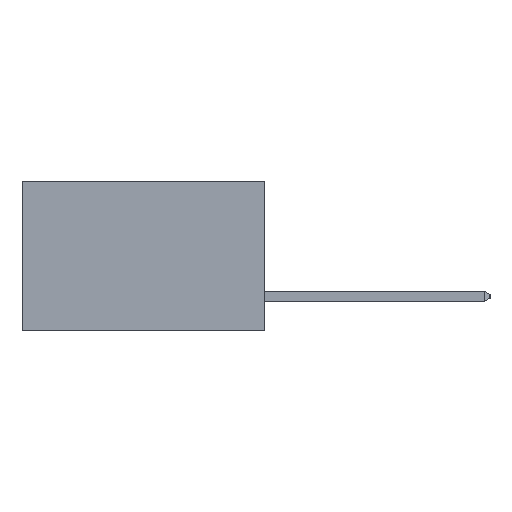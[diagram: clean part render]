
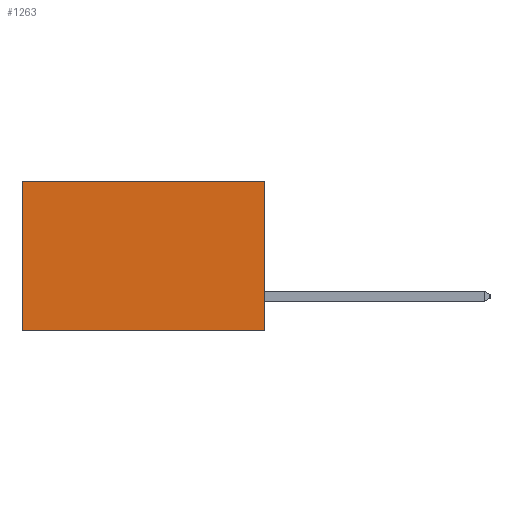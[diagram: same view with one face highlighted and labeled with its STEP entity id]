
A CAD part, left-side view. The second image highlights one B-rep face of the part: STEP entity #1263.
In plain terms, the highlighted planar face has unit normal (-1, 0, 0).
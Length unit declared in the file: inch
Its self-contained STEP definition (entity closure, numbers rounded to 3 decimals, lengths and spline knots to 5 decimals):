
#1263 = ADVANCED_FACE ( 'NONE', ( #21789 ), #15451, .F. ) ;
#1302 = EDGE_LOOP ( 'NONE', ( #18955, #6433, #19054, #21128 ) ) ;
#1307 = EDGE_CURVE ( 'NONE', #15340, #2263, #1640, .T. ) ;
#1640 = LINE ( 'NONE', #10880, #11262 ) ;
#1759 = CARTESIAN_POINT ( 'NONE',  ( 0.2615, 0.6, -0.37 ) ) ;
#2263 = VERTEX_POINT ( 'NONE', #3046 ) ;
#2740 = VECTOR ( 'NONE', #22175, 39.37008 ) ;
#3046 = CARTESIAN_POINT ( 'NONE',  ( 0.2615, 0.6, 0. ) ) ;
#3265 = CARTESIAN_POINT ( 'NONE',  ( 0.2615, 0.6, -0.37 ) ) ;
#4003 = LINE ( 'NONE', #20665, #22865 ) ;
#6433 = ORIENTED_EDGE ( 'NONE', *, *, #14882, .F. ) ;
#8589 = VECTOR ( 'NONE', #19528, 39.37008 ) ;
#10880 = CARTESIAN_POINT ( 'NONE',  ( 0.2615, 0., 0. ) ) ;
#10926 = CARTESIAN_POINT ( 'NONE',  ( 0.2615, 0., 0. ) ) ;
#11262 = VECTOR ( 'NONE', #13035, 39.37008 ) ;
#11428 = CARTESIAN_POINT ( 'NONE',  ( 0.2615, 0., -0.37 ) ) ;
#13035 = DIRECTION ( 'NONE',  ( 0., 1., 0. ) ) ;
#14216 = DIRECTION ( 'NONE',  ( 1., 0., 0. ) ) ;
#14882 = EDGE_CURVE ( 'NONE', #14916, #16942, #4003, .T. ) ;
#14916 = VERTEX_POINT ( 'NONE', #11428 ) ;
#15318 = EDGE_CURVE ( 'NONE', #2263, #16942, #22838, .T. ) ;
#15340 = VERTEX_POINT ( 'NONE', #10926 ) ;
#15451 = PLANE ( 'NONE',  #23862 ) ;
#16942 = VERTEX_POINT ( 'NONE', #1759 ) ;
#18955 = ORIENTED_EDGE ( 'NONE', *, *, #15318, .T. ) ;
#19035 = EDGE_CURVE ( 'NONE', #15340, #14916, #23472, .T. ) ;
#19054 = ORIENTED_EDGE ( 'NONE', *, *, #19035, .F. ) ;
#19089 = DIRECTION ( 'NONE',  ( 0., 0., -1. ) ) ;
#19528 = DIRECTION ( 'NONE',  ( 0., 0., -1. ) ) ;
#20665 = CARTESIAN_POINT ( 'NONE',  ( 0.2615, 0., -0.37 ) ) ;
#21128 = ORIENTED_EDGE ( 'NONE', *, *, #1307, .T. ) ;
#21311 = CARTESIAN_POINT ( 'NONE',  ( 0.2615, 0., -0.37 ) ) ;
#21789 = FACE_OUTER_BOUND ( 'NONE', #1302, .T. ) ;
#22175 = DIRECTION ( 'NONE',  ( 0., 0., -1. ) ) ;
#22509 = DIRECTION ( 'NONE',  ( 0., 1., 0. ) ) ;
#22838 = LINE ( 'NONE', #3265, #2740 ) ;
#22865 = VECTOR ( 'NONE', #22509, 39.37008 ) ;
#23472 = LINE ( 'NONE', #21311, #8589 ) ;
#23721 = CARTESIAN_POINT ( 'NONE',  ( 0.2615, 0., -0.37 ) ) ;
#23862 = AXIS2_PLACEMENT_3D ( 'NONE', #23721, #14216, #19089 ) ;
